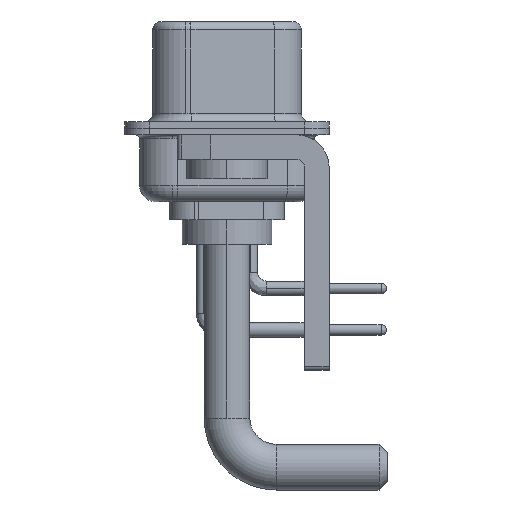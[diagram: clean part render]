
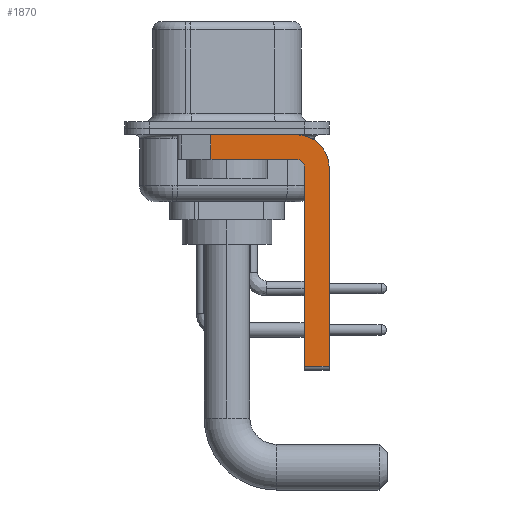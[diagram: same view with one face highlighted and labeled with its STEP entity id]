
A CAD part, left-side view. The second image highlights one B-rep face of the part: STEP entity #1870.
In plain terms, the highlighted planar face has unit normal (-1, 0, 0).
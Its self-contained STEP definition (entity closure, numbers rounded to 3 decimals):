
#949 = AXIS2_PLACEMENT_3D ( 'NONE', #13832, #18220, #7383 ) ;
#1128 = VERTEX_POINT ( 'NONE', #15137 ) ;
#1616 = AXIS2_PLACEMENT_3D ( 'NONE', #27601, #26791, #10993 ) ;
#1870 = ADVANCED_FACE ( 'NONE', ( #27304 ), #18271, .F. ) ;
#1898 = CARTESIAN_POINT ( 'NONE',  ( -2.9, -4.25, -14.55 ) ) ;
#2037 = CARTESIAN_POINT ( 'NONE',  ( -2.9, 0.978, -1.9 ) ) ;
#2059 = CARTESIAN_POINT ( 'NONE',  ( -2.9, -4.75, -14.8 ) ) ;
#2466 = CARTESIAN_POINT ( 'NONE',  ( -2.9, -4.25, -1.9 ) ) ;
#2927 = ORIENTED_EDGE ( 'NONE', *, *, #10109, .F. ) ;
#3463 = CARTESIAN_POINT ( 'NONE',  ( -2.9, -6.25, -2.4 ) ) ;
#3723 = ORIENTED_EDGE ( 'NONE', *, *, #8502, .F. ) ;
#4988 = DIRECTION ( 'NONE',  ( 1., 0., 0. ) ) ;
#5045 = DIRECTION ( 'NONE',  ( 0., 0., -1. ) ) ;
#5931 = LINE ( 'NONE', #3463, #7054 ) ;
#5948 = EDGE_CURVE ( 'NONE', #8752, #25699, #14219, .T. ) ;
#5983 = DIRECTION ( 'NONE',  ( 0., -1., 0. ) ) ;
#7054 = VECTOR ( 'NONE', #7823, 1000. ) ;
#7209 = CARTESIAN_POINT ( 'NONE',  ( -2.9, 0.978, -1.9 ) ) ;
#7383 = DIRECTION ( 'NONE',  ( 0., 0., -1. ) ) ;
#7459 = CIRCLE ( 'NONE', #949, 2. ) ;
#7823 = DIRECTION ( 'NONE',  ( 0., 0., -1. ) ) ;
#7865 = ORIENTED_EDGE ( 'NONE', *, *, #17768, .F. ) ;
#8116 = CIRCLE ( 'NONE', #1616, 0.5 ) ;
#8502 = EDGE_CURVE ( 'NONE', #1128, #26729, #7459, .T. ) ;
#8752 = VERTEX_POINT ( 'NONE', #21129 ) ;
#9059 = ORIENTED_EDGE ( 'NONE', *, *, #13903, .F. ) ;
#10109 = EDGE_CURVE ( 'NONE', #26729, #17932, #5931, .T. ) ;
#10158 = LINE ( 'NONE', #16590, #21981 ) ;
#10915 = DIRECTION ( 'NONE',  ( 0., 1., 0. ) ) ;
#10993 = DIRECTION ( 'NONE',  ( 0., 0., 1. ) ) ;
#11320 = CARTESIAN_POINT ( 'NONE',  ( -2.9, -4.75, -2.4 ) ) ;
#11547 = CARTESIAN_POINT ( 'NONE',  ( -2.9, -4.25, -2.4 ) ) ;
#11705 = CARTESIAN_POINT ( 'NONE',  ( -2.9, -4.75, -14.55 ) ) ;
#11947 = ORIENTED_EDGE ( 'NONE', *, *, #5948, .T. ) ;
#12713 = LINE ( 'NONE', #2059, #23232 ) ;
#13041 = CARTESIAN_POINT ( 'NONE',  ( -2.9, -6.25, -2.4 ) ) ;
#13348 = VECTOR ( 'NONE', #5045, 1000. ) ;
#13415 = LINE ( 'NONE', #2466, #26914 ) ;
#13832 = CARTESIAN_POINT ( 'NONE',  ( -2.9, -4.25, -2.4 ) ) ;
#13903 = EDGE_CURVE ( 'NONE', #17568, #22947, #12713, .T. ) ;
#14219 = LINE ( 'NONE', #7209, #13348 ) ;
#14556 = DIRECTION ( 'NONE',  ( 0., -1., 0. ) ) ;
#15137 = CARTESIAN_POINT ( 'NONE',  ( -2.9, -4.25, -0.4 ) ) ;
#16590 = CARTESIAN_POINT ( 'NONE',  ( -2.9, 3., -0.4 ) ) ;
#17066 = LINE ( 'NONE', #1898, #23101 ) ;
#17518 = DIRECTION ( 'NONE',  ( 0., 0., 1. ) ) ;
#17568 = VERTEX_POINT ( 'NONE', #11705 ) ;
#17691 = CARTESIAN_POINT ( 'NONE',  ( -2.9, -4.25, -1.9 ) ) ;
#17768 = EDGE_CURVE ( 'NONE', #22947, #21471, #8116, .T. ) ;
#17932 = VERTEX_POINT ( 'NONE', #26354 ) ;
#18220 = DIRECTION ( 'NONE',  ( 1., 0., 0. ) ) ;
#18271 = PLANE ( 'NONE',  #27618 ) ;
#18669 = EDGE_CURVE ( 'NONE', #17568, #17932, #17066, .T. ) ;
#19756 = ORIENTED_EDGE ( 'NONE', *, *, #25839, .F. ) ;
#20151 = ORIENTED_EDGE ( 'NONE', *, *, #20503, .F. ) ;
#20473 = DIRECTION ( 'NONE',  ( 0., 0., -1. ) ) ;
#20503 = EDGE_CURVE ( 'NONE', #21471, #25699, #13415, .T. ) ;
#21129 = CARTESIAN_POINT ( 'NONE',  ( -2.9, 0.978, -0.4 ) ) ;
#21471 = VERTEX_POINT ( 'NONE', #17691 ) ;
#21981 = VECTOR ( 'NONE', #14556, 1000. ) ;
#22947 = VERTEX_POINT ( 'NONE', #11320 ) ;
#23101 = VECTOR ( 'NONE', #5983, 1000. ) ;
#23232 = VECTOR ( 'NONE', #17518, 1000. ) ;
#25168 = EDGE_LOOP ( 'NONE', ( #19756, #11947, #20151, #7865, #9059, #27173, #2927, #3723 ) ) ;
#25699 = VERTEX_POINT ( 'NONE', #2037 ) ;
#25839 = EDGE_CURVE ( 'NONE', #8752, #1128, #10158, .T. ) ;
#26354 = CARTESIAN_POINT ( 'NONE',  ( -2.9, -6.25, -14.55 ) ) ;
#26729 = VERTEX_POINT ( 'NONE', #13041 ) ;
#26791 = DIRECTION ( 'NONE',  ( -1., 0., 0. ) ) ;
#26914 = VECTOR ( 'NONE', #10915, 1000. ) ;
#27173 = ORIENTED_EDGE ( 'NONE', *, *, #18669, .T. ) ;
#27304 = FACE_OUTER_BOUND ( 'NONE', #25168, .T. ) ;
#27601 = CARTESIAN_POINT ( 'NONE',  ( -2.9, -4.25, -2.4 ) ) ;
#27618 = AXIS2_PLACEMENT_3D ( 'NONE', #11547, #4988, #20473 ) ;
